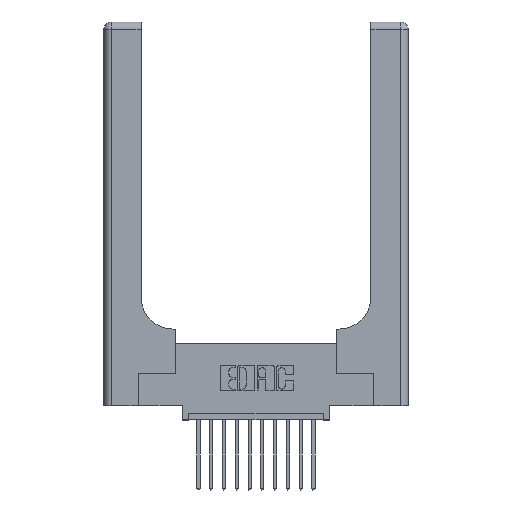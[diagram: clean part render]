
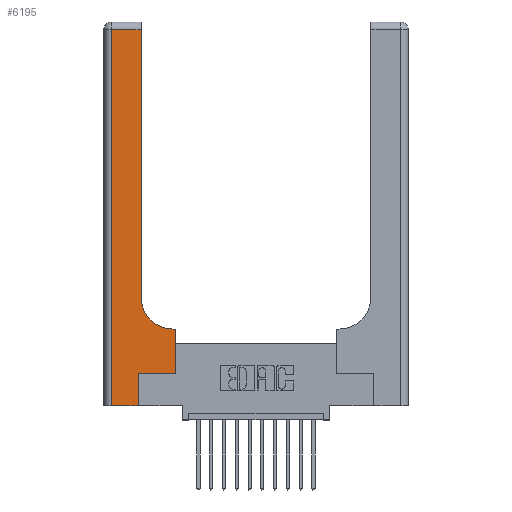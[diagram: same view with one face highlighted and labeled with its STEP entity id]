
A CAD part, top view. The second image highlights one B-rep face of the part: STEP entity #6195.
In plain terms, the highlighted planar face has unit normal (0, 0, 1).
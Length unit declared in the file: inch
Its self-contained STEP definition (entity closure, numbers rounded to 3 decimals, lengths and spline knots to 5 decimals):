
#361 = EDGE_CURVE ( 'NONE', #11542, #8258, #16048, .T. ) ;
#883 = VERTEX_POINT ( 'NONE', #2255 ) ;
#1229 = DIRECTION ( 'NONE',  ( 1., 0., 0. ) ) ;
#1285 = ORIENTED_EDGE ( 'NONE', *, *, #361, .T. ) ;
#1608 = AXIS2_PLACEMENT_3D ( 'NONE', #14860, #4529, #16478 ) ;
#1663 = CARTESIAN_POINT ( 'NONE',  ( 0.5415, 0.85, 0.37 ) ) ;
#1762 = CARTESIAN_POINT ( 'NONE',  ( 0.06, 2.94, 0.37 ) ) ;
#1850 = VERTEX_POINT ( 'NONE', #10050 ) ;
#1975 = LINE ( 'NONE', #7238, #15044 ) ;
#2255 = CARTESIAN_POINT ( 'NONE',  ( 0.5585, 0.25, 0.37 ) ) ;
#2330 = CARTESIAN_POINT ( 'NONE',  ( 0.2915, 2.94, 0.37 ) ) ;
#3173 = ORIENTED_EDGE ( 'NONE', *, *, #15869, .T. ) ;
#3375 = EDGE_CURVE ( 'NONE', #13945, #14763, #4334, .T. ) ;
#4116 = VECTOR ( 'NONE', #12885, 39.37008 ) ;
#4208 = VECTOR ( 'NONE', #4810, 39.37008 ) ;
#4304 = DIRECTION ( 'NONE',  ( 1., 0., 0. ) ) ;
#4334 = LINE ( 'NONE', #11538, #4116 ) ;
#4529 = DIRECTION ( 'NONE',  ( 0., 0., -1. ) ) ;
#4796 = EDGE_CURVE ( 'NONE', #14876, #10977, #1975, .T. ) ;
#4810 = DIRECTION ( 'NONE',  ( 0., 1., 0. ) ) ;
#5045 = VECTOR ( 'NONE', #9506, 39.37008 ) ;
#5248 = ORIENTED_EDGE ( 'NONE', *, *, #11789, .T. ) ;
#5445 = PLANE ( 'NONE',  #1608 ) ;
#5471 = VECTOR ( 'NONE', #16826, 39.37008 ) ;
#5684 = LINE ( 'NONE', #9026, #5471 ) ;
#5943 = DIRECTION ( 'NONE',  ( -1., 0., 0. ) ) ;
#6008 = ORIENTED_EDGE ( 'NONE', *, *, #14802, .T. ) ;
#6195 = ADVANCED_FACE ( 'NONE', ( #13525 ), #5445, .F. ) ;
#6453 = EDGE_CURVE ( 'NONE', #1850, #13945, #6616, .T. ) ;
#6616 = CIRCLE ( 'NONE', #11127, 0.25 ) ;
#6653 = CARTESIAN_POINT ( 'NONE',  ( 0.269, 0.25, 0.37 ) ) ;
#7204 = VECTOR ( 'NONE', #15911, 39.37008 ) ;
#7238 = CARTESIAN_POINT ( 'NONE',  ( 0.06, 3., 0.37 ) ) ;
#8104 = CARTESIAN_POINT ( 'NONE',  ( 0.5585, 0.25, 0.37 ) ) ;
#8258 = VERTEX_POINT ( 'NONE', #8626 ) ;
#8499 = CARTESIAN_POINT ( 'NONE',  ( 0.06, 0., 0.37 ) ) ;
#8576 = DIRECTION ( 'NONE',  ( 0., -1., 0. ) ) ;
#8626 = CARTESIAN_POINT ( 'NONE',  ( 0.269, 0.25, 0.37 ) ) ;
#8697 = LINE ( 'NONE', #9731, #9986 ) ;
#9026 = CARTESIAN_POINT ( 'NONE',  ( 0., 0., 0.37 ) ) ;
#9506 = DIRECTION ( 'NONE',  ( 0., 1., 0. ) ) ;
#9689 = ORIENTED_EDGE ( 'NONE', *, *, #3375, .T. ) ;
#9731 = CARTESIAN_POINT ( 'NONE',  ( 0., 2.94, 0.37 ) ) ;
#9986 = VECTOR ( 'NONE', #5943, 39.37008 ) ;
#10050 = CARTESIAN_POINT ( 'NONE',  ( 0.5415, 0.6, 0.37 ) ) ;
#10185 = CARTESIAN_POINT ( 'NONE',  ( 0.2915, 0.85, 0.37 ) ) ;
#10559 = ORIENTED_EDGE ( 'NONE', *, *, #12604, .T. ) ;
#10770 = LINE ( 'NONE', #14805, #7204 ) ;
#10977 = VERTEX_POINT ( 'NONE', #8499 ) ;
#11117 = ORIENTED_EDGE ( 'NONE', *, *, #16613, .T. ) ;
#11127 = AXIS2_PLACEMENT_3D ( 'NONE', #1663, #16142, #4304 ) ;
#11538 = CARTESIAN_POINT ( 'NONE',  ( 0.2915, 3., 0.37 ) ) ;
#11542 = VERTEX_POINT ( 'NONE', #16644 ) ;
#11778 = VECTOR ( 'NONE', #1229, 39.37008 ) ;
#11789 = EDGE_CURVE ( 'NONE', #13117, #1850, #10770, .T. ) ;
#12195 = ORIENTED_EDGE ( 'NONE', *, *, #4796, .T. ) ;
#12604 = EDGE_CURVE ( 'NONE', #8258, #883, #16778, .T. ) ;
#12712 = CARTESIAN_POINT ( 'NONE',  ( 0.269, 0., 0.37 ) ) ;
#12885 = DIRECTION ( 'NONE',  ( 0., 1., 0. ) ) ;
#12962 = ORIENTED_EDGE ( 'NONE', *, *, #6453, .T. ) ;
#13117 = VERTEX_POINT ( 'NONE', #13546 ) ;
#13479 = EDGE_LOOP ( 'NONE', ( #9689, #11117, #12195, #6008, #1285, #10559, #3173, #5248, #12962 ) ) ;
#13525 = FACE_OUTER_BOUND ( 'NONE', #13479, .T. ) ;
#13546 = CARTESIAN_POINT ( 'NONE',  ( 0.5585, 0.6, 0.37 ) ) ;
#13945 = VERTEX_POINT ( 'NONE', #10185 ) ;
#14002 = LINE ( 'NONE', #8104, #5045 ) ;
#14763 = VERTEX_POINT ( 'NONE', #2330 ) ;
#14802 = EDGE_CURVE ( 'NONE', #10977, #11542, #5684, .T. ) ;
#14805 = CARTESIAN_POINT ( 'NONE',  ( 0.2915, 0.6, 0.37 ) ) ;
#14860 = CARTESIAN_POINT ( 'NONE',  ( 0., 3., 0.37 ) ) ;
#14876 = VERTEX_POINT ( 'NONE', #1762 ) ;
#15044 = VECTOR ( 'NONE', #8576, 39.37008 ) ;
#15869 = EDGE_CURVE ( 'NONE', #883, #13117, #14002, .T. ) ;
#15911 = DIRECTION ( 'NONE',  ( -1., 0., 0. ) ) ;
#16048 = LINE ( 'NONE', #12712, #4208 ) ;
#16142 = DIRECTION ( 'NONE',  ( 0., 0., -1. ) ) ;
#16478 = DIRECTION ( 'NONE',  ( -1., 0., 0. ) ) ;
#16613 = EDGE_CURVE ( 'NONE', #14763, #14876, #8697, .T. ) ;
#16644 = CARTESIAN_POINT ( 'NONE',  ( 0.269, 0., 0.37 ) ) ;
#16778 = LINE ( 'NONE', #6653, #11778 ) ;
#16826 = DIRECTION ( 'NONE',  ( 1., 0., 0. ) ) ;
